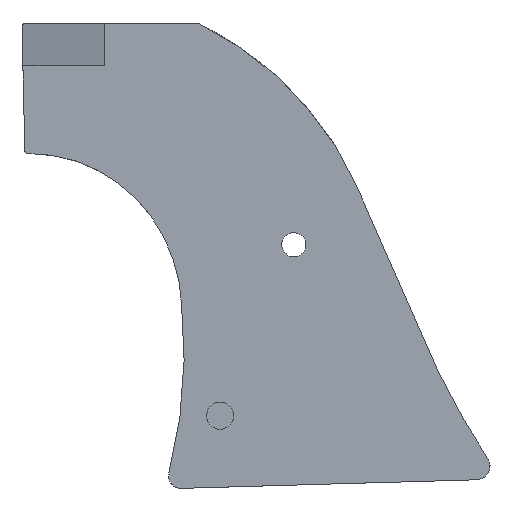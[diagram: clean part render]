
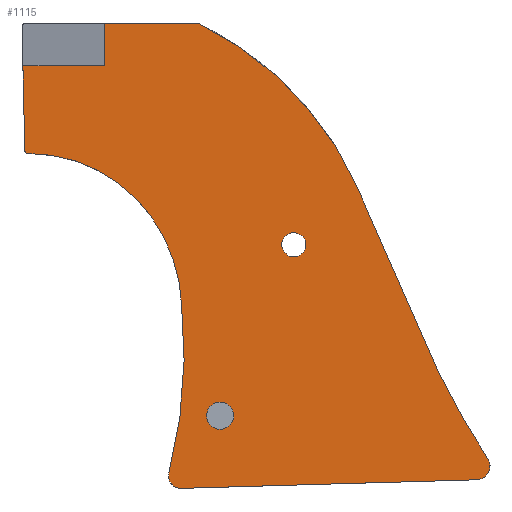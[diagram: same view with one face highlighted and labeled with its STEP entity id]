
A CAD part, left-side view. The second image highlights one B-rep face of the part: STEP entity #1115.
In plain terms, the highlighted planar face has unit normal (-1, 0, 0).
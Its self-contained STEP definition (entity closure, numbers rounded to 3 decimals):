
#91=LINE('',#2046,#167);
#108=LINE('',#2399,#184);
#112=LINE('',#2409,#188);
#113=LINE('',#2412,#189);
#114=LINE('',#2414,#190);
#115=LINE('',#2417,#191);
#116=LINE('',#2419,#192);
#117=LINE('',#2420,#193);
#167=VECTOR('',#1437,10.);
#184=VECTOR('',#1520,10.);
#188=VECTOR('',#1528,10.);
#189=VECTOR('',#1531,10.);
#190=VECTOR('',#1532,10.);
#191=VECTOR('',#1535,10.);
#192=VECTOR('',#1536,10.);
#193=VECTOR('',#1537,10.);
#244=FACE_BOUND('',#373,.T.);
#245=FACE_BOUND('',#374,.T.);
#295=FACE_OUTER_BOUND('',#372,.T.);
#372=EDGE_LOOP('',(#924,#925,#926,#927,#928,#929,#930,#931,#932,#933,#934,
#935,#936,#937,#938,#939,#940,#941));
#373=EDGE_LOOP('',(#942));
#374=EDGE_LOOP('',(#943));
#416=CIRCLE('',#1192,2.);
#423=CIRCLE('',#1203,2.);
#424=CIRCLE('',#1205,78.627);
#432=CIRCLE('',#1224,0.5);
#439=CIRCLE('',#1234,0.5);
#444=CIRCLE('',#1242,25.021);
#445=CIRCLE('',#1245,2.096);
#446=CIRCLE('',#1246,2.353);
#447=CIRCLE('',#1247,54.617);
#448=CIRCLE('',#1248,27.174);
#449=CIRCLE('',#1249,2.25);
#450=CIRCLE('',#1250,2.);
#489=VERTEX_POINT('',#1719);
#490=VERTEX_POINT('',#1720);
#501=VERTEX_POINT('',#2015);
#502=VERTEX_POINT('',#2016);
#503=VERTEX_POINT('',#2021);
#506=VERTEX_POINT('',#2044);
#521=VERTEX_POINT('',#2254);
#522=VERTEX_POINT('',#2255);
#534=VERTEX_POINT('',#2381);
#535=VERTEX_POINT('',#2382);
#537=VERTEX_POINT('',#2394);
#538=VERTEX_POINT('',#2398);
#541=VERTEX_POINT('',#2406);
#542=VERTEX_POINT('',#2408);
#543=VERTEX_POINT('',#2411);
#544=VERTEX_POINT('',#2413);
#545=VERTEX_POINT('',#2416);
#546=VERTEX_POINT('',#2418);
#547=VERTEX_POINT('',#2422);
#548=VERTEX_POINT('',#2424);
#601=EDGE_CURVE('',#489,#490,#416,.T.);
#619=EDGE_CURVE('',#501,#502,#423,.T.);
#622=EDGE_CURVE('',#489,#503,#424,.T.);
#629=EDGE_CURVE('',#506,#502,#91,.T.);
#652=EDGE_CURVE('',#521,#522,#432,.T.);
#669=EDGE_CURVE('',#534,#535,#439,.T.);
#677=EDGE_CURVE('',#537,#522,#444,.T.);
#678=EDGE_CURVE('',#521,#538,#108,.T.);
#682=EDGE_CURVE('',#541,#490,#445,.T.);
#683=EDGE_CURVE('',#542,#541,#112,.T.);
#684=EDGE_CURVE('',#501,#542,#446,.T.);
#685=EDGE_CURVE('',#543,#506,#113,.T.);
#686=EDGE_CURVE('',#544,#543,#114,.T.);
#687=EDGE_CURVE('',#534,#544,#447,.T.);
#688=EDGE_CURVE('',#545,#535,#115,.T.);
#689=EDGE_CURVE('',#546,#545,#116,.T.);
#690=EDGE_CURVE('',#538,#546,#117,.T.);
#691=EDGE_CURVE('',#503,#537,#448,.T.);
#692=EDGE_CURVE('',#547,#547,#449,.T.);
#693=EDGE_CURVE('',#548,#548,#450,.T.);
#924=ORIENTED_EDGE('',*,*,#601,.T.);
#925=ORIENTED_EDGE('',*,*,#682,.F.);
#926=ORIENTED_EDGE('',*,*,#683,.F.);
#927=ORIENTED_EDGE('',*,*,#684,.F.);
#928=ORIENTED_EDGE('',*,*,#619,.T.);
#929=ORIENTED_EDGE('',*,*,#629,.F.);
#930=ORIENTED_EDGE('',*,*,#685,.F.);
#931=ORIENTED_EDGE('',*,*,#686,.F.);
#932=ORIENTED_EDGE('',*,*,#687,.F.);
#933=ORIENTED_EDGE('',*,*,#669,.T.);
#934=ORIENTED_EDGE('',*,*,#688,.F.);
#935=ORIENTED_EDGE('',*,*,#689,.F.);
#936=ORIENTED_EDGE('',*,*,#690,.F.);
#937=ORIENTED_EDGE('',*,*,#678,.F.);
#938=ORIENTED_EDGE('',*,*,#652,.T.);
#939=ORIENTED_EDGE('',*,*,#677,.F.);
#940=ORIENTED_EDGE('',*,*,#691,.F.);
#941=ORIENTED_EDGE('',*,*,#622,.F.);
#942=ORIENTED_EDGE('',*,*,#692,.F.);
#943=ORIENTED_EDGE('',*,*,#693,.F.);
#1056=PLANE('',#1244);
#1115=ADVANCED_FACE('',(#295,#244,#245),#1056,.F.);
#1192=AXIS2_PLACEMENT_3D('',#1721,#1391,#1392);
#1203=AXIS2_PLACEMENT_3D('',#2017,#1416,#1417);
#1205=AXIS2_PLACEMENT_3D('',#2022,#1422,#1423);
#1224=AXIS2_PLACEMENT_3D('',#2256,#1471,#1472);
#1234=AXIS2_PLACEMENT_3D('',#2383,#1497,#1498);
#1242=AXIS2_PLACEMENT_3D('',#2396,#1516,#1517);
#1244=AXIS2_PLACEMENT_3D('',#2405,#1524,#1525);
#1245=AXIS2_PLACEMENT_3D('',#2407,#1526,#1527);
#1246=AXIS2_PLACEMENT_3D('',#2410,#1529,#1530);
#1247=AXIS2_PLACEMENT_3D('',#2415,#1533,#1534);
#1248=AXIS2_PLACEMENT_3D('',#2421,#1538,#1539);
#1249=AXIS2_PLACEMENT_3D('',#2423,#1540,#1541);
#1250=AXIS2_PLACEMENT_3D('',#2425,#1542,#1543);
#1391=DIRECTION('center_axis',(-1.,0.,0.));
#1392=DIRECTION('ref_axis',(0.,0.999,0.048));
#1416=DIRECTION('center_axis',(-1.,0.,0.));
#1417=DIRECTION('ref_axis',(0.,-0.961,0.276));
#1422=DIRECTION('center_axis',(-1.,0.,0.));
#1423=DIRECTION('ref_axis',(0.,-0.995,0.104));
#1437=DIRECTION('',(0.,-0.523,-0.852));
#1471=DIRECTION('center_axis',(-1.,0.,0.));
#1472=DIRECTION('ref_axis',(0.,0.698,-0.716));
#1497=DIRECTION('center_axis',(-1.,0.,0.));
#1498=DIRECTION('ref_axis',(0.,-0.223,0.975));
#1516=DIRECTION('center_axis',(-1.,0.,0.));
#1517=DIRECTION('ref_axis',(0.,0.023,1.));
#1520=DIRECTION('',(0.,0.023,1.));
#1524=DIRECTION('center_axis',(1.,0.,0.));
#1525=DIRECTION('ref_axis',(0.,1.,0.));
#1526=DIRECTION('center_axis',(1.,0.,0.));
#1527=DIRECTION('ref_axis',(0.,-0.029,-1.));
#1528=DIRECTION('',(0.,1.,-0.029));
#1529=DIRECTION('center_axis',(1.,0.,0.));
#1530=DIRECTION('ref_axis',(0.,-0.942,0.336));
#1531=DIRECTION('',(0.,-0.469,-0.883));
#1532=DIRECTION('',(0.,-0.403,-0.915));
#1533=DIRECTION('center_axis',(1.,0.,0.));
#1534=DIRECTION('ref_axis',(0.,-0.433,0.901));
#1535=DIRECTION('',(0.,-1.,0.));
#1536=DIRECTION('',(0.,0.,1.));
#1537=DIRECTION('',(0.,-1.,0.));
#1538=DIRECTION('center_axis',(-1.,0.,0.));
#1539=DIRECTION('ref_axis',(0.,-0.814,0.58));
#1540=DIRECTION('center_axis',(-1.,0.,0.));
#1541=DIRECTION('ref_axis',(0.,-1.,0.));
#1542=DIRECTION('center_axis',(-1.,0.,0.));
#1543=DIRECTION('ref_axis',(0.,-1.,0.));
#1719=CARTESIAN_POINT('',(3.808,-12.899,-414.573));
#1720=CARTESIAN_POINT('',(3.808,-12.859,-415.392));
#1721=CARTESIAN_POINT('Origin',(3.808,-14.834,-415.077));
#2015=CARTESIAN_POINT('',(3.808,-66.103,-413.365));
#2016=CARTESIAN_POINT('',(3.808,-65.807,-412.336));
#2017=CARTESIAN_POINT('Origin',(3.808,-64.103,-413.381));
#2021=CARTESIAN_POINT('',(3.808,-15.002,-386.617));
#2022=CARTESIAN_POINT('Origin',(3.808,63.199,-394.792));
#2044=CARTESIAN_POINT('',(3.808,-61.669,-405.59));
#2046=CARTESIAN_POINT('',(3.808,-61.669,-405.59));
#2254=CARTESIAN_POINT('',(3.808,10.978,-361.177));
#2255=CARTESIAN_POINT('',(3.808,10.477,-361.666));
#2256=CARTESIAN_POINT('Origin',(3.808,10.478,-361.166));
#2381=CARTESIAN_POINT('',(3.808,-17.907,-340.205));
#2382=CARTESIAN_POINT('',(3.808,-17.689,-340.155));
#2383=CARTESIAN_POINT('Origin',(3.808,-17.689,-340.655));
#2394=CARTESIAN_POINT('',(3.808,-9.99,-372.167));
#2396=CARTESIAN_POINT('Origin',(3.808,10.387,-386.686));
#2398=CARTESIAN_POINT('',(3.808,11.295,-347.158));
#2399=CARTESIAN_POINT('',(3.808,11.454,-340.155));
#2405=CARTESIAN_POINT('Origin',(3.808,-27.324,-378.656));
#2406=CARTESIAN_POINT('',(3.808,-14.99,-417.157));
#2407=CARTESIAN_POINT('Origin',(3.808,-14.929,-415.061));
#2408=CARTESIAN_POINT('',(3.808,-63.818,-415.737));
#2409=CARTESIAN_POINT('',(3.808,-63.818,-415.737));
#2410=CARTESIAN_POINT('Origin',(3.808,-63.749,-413.384));
#2411=CARTESIAN_POINT('',(3.808,-57.611,-397.958));
#2412=CARTESIAN_POINT('',(3.808,-57.611,-397.958));
#2413=CARTESIAN_POINT('',(3.808,-44.15,-367.383));
#2414=CARTESIAN_POINT('',(3.808,-44.15,-367.383));
#2415=CARTESIAN_POINT('Origin',(3.808,5.837,-389.391));
#2416=CARTESIAN_POINT('',(3.808,-2.225,-340.155));
#2417=CARTESIAN_POINT('',(3.808,11.454,-340.155));
#2418=CARTESIAN_POINT('',(3.808,-2.225,-347.158));
#2419=CARTESIAN_POINT('',(3.808,-2.225,-362.907));
#2420=CARTESIAN_POINT('',(3.808,-8.015,-347.158));
#2421=CARTESIAN_POINT('Origin',(3.808,12.141,-387.936));
#2422=CARTESIAN_POINT('',(3.808,-19.129,-405.119));
#2423=CARTESIAN_POINT('Origin',(3.808,-21.379,-405.119));
#2424=CARTESIAN_POINT('',(3.808,-31.595,-376.79));
#2425=CARTESIAN_POINT('Origin',(3.808,-33.595,-376.79));
